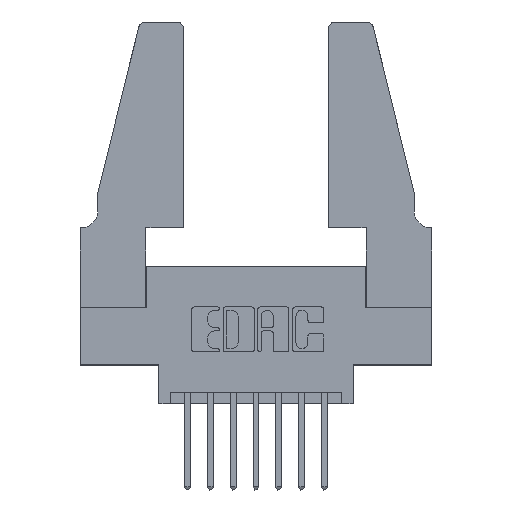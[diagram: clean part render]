
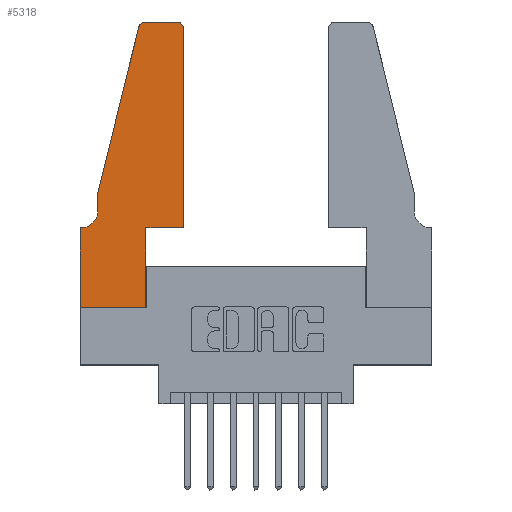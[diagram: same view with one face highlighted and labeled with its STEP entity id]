
A CAD part, top view. The second image highlights one B-rep face of the part: STEP entity #5318.
In plain terms, the highlighted planar face has unit normal (0, 0, 1).
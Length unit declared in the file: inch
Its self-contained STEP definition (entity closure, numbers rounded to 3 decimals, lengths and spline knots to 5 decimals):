
#15 = CARTESIAN_POINT ( 'NONE',  ( 0., 0., 0.37 ) ) ;
#160 = EDGE_CURVE ( 'NONE', #8481, #1776, #9997, .T. ) ;
#842 = CIRCLE ( 'NONE', #3955, 0.03 ) ;
#1019 = ORIENTED_EDGE ( 'NONE', *, *, #10509, .T. ) ;
#1210 = CARTESIAN_POINT ( 'NONE',  ( 0.0755, 0.35, 0.37 ) ) ;
#1450 = ORIENTED_EDGE ( 'NONE', *, *, #7952, .T. ) ;
#1519 = ORIENTED_EDGE ( 'NONE', *, *, #4496, .T. ) ;
#1522 = VECTOR ( 'NONE', #3505, 39.37008 ) ;
#1612 = CARTESIAN_POINT ( 'NONE',  ( 0.2605, 1.25, 0.37 ) ) ;
#1715 = VERTEX_POINT ( 'NONE', #7712 ) ;
#1736 = EDGE_CURVE ( 'NONE', #5225, #1715, #4341, .T. ) ;
#1776 = VERTEX_POINT ( 'NONE', #3939 ) ;
#1782 = VECTOR ( 'NONE', #1790, 39.37008 ) ;
#1790 = DIRECTION ( 'NONE',  ( 0., -1., 0. ) ) ;
#1913 = PLANE ( 'NONE',  #7989 ) ;
#1926 = VERTEX_POINT ( 'NONE', #6098 ) ;
#2149 = ORIENTED_EDGE ( 'NONE', *, *, #1736, .T. ) ;
#2247 = CARTESIAN_POINT ( 'NONE',  ( 0., 0.35, 0.37 ) ) ;
#2248 = CARTESIAN_POINT ( 'NONE',  ( 0.0055, 0.35, 0.37 ) ) ;
#2480 = LINE ( 'NONE', #1612, #10797 ) ;
#2483 = ORIENTED_EDGE ( 'NONE', *, *, #7764, .T. ) ;
#2569 = CARTESIAN_POINT ( 'NONE',  ( 0.2865, 0.35, 0.37 ) ) ;
#2585 = ORIENTED_EDGE ( 'NONE', *, *, #12018, .T. ) ;
#2682 = VERTEX_POINT ( 'NONE', #10618 ) ;
#2702 = CARTESIAN_POINT ( 'NONE',  ( 0.0055, 0.42, 0.37 ) ) ;
#2733 = ORIENTED_EDGE ( 'NONE', *, *, #11453, .T. ) ;
#3236 = ORIENTED_EDGE ( 'NONE', *, *, #4922, .T. ) ;
#3317 = EDGE_LOOP ( 'NONE', ( #8560, #2483, #6055, #1019, #2733, #10747, #2149, #1450, #2585, #3541, #1519, #3236 ) ) ;
#3361 = VERTEX_POINT ( 'NONE', #2248 ) ;
#3505 = DIRECTION ( 'NONE',  ( -0.239, -0.971, 0. ) ) ;
#3541 = ORIENTED_EDGE ( 'NONE', *, *, #160, .T. ) ;
#3655 = VECTOR ( 'NONE', #4179, 39.37008 ) ;
#3939 = CARTESIAN_POINT ( 'NONE',  ( 0.4505, 0.35, 0.37 ) ) ;
#3954 = CARTESIAN_POINT ( 'NONE',  ( 0.4205, 1.25, 0.37 ) ) ;
#3955 = AXIS2_PLACEMENT_3D ( 'NONE', #11658, #5882, #9820 ) ;
#4040 = VECTOR ( 'NONE', #4442, 39.37008 ) ;
#4054 = LINE ( 'NONE', #12157, #10863 ) ;
#4137 = VERTEX_POINT ( 'NONE', #4592 ) ;
#4179 = DIRECTION ( 'NONE',  ( -1., 0., 0. ) ) ;
#4250 = VERTEX_POINT ( 'NONE', #11730 ) ;
#4341 = LINE ( 'NONE', #15, #1782 ) ;
#4442 = DIRECTION ( 'NONE',  ( 1., 0., 0. ) ) ;
#4496 = EDGE_CURVE ( 'NONE', #1776, #2682, #7743, .T. ) ;
#4592 = CARTESIAN_POINT ( 'NONE',  ( 0.0755, 0.42, 0.37 ) ) ;
#4639 = DIRECTION ( 'NONE',  ( 0., 1., 0. ) ) ;
#4673 = EDGE_CURVE ( 'NONE', #6773, #4250, #2480, .T. ) ;
#4731 = CARTESIAN_POINT ( 'NONE',  ( 0.284, 1.22, 0.37 ) ) ;
#4922 = EDGE_CURVE ( 'NONE', #2682, #6773, #842, .T. ) ;
#5225 = VERTEX_POINT ( 'NONE', #2247 ) ;
#5318 = ADVANCED_FACE ( 'NONE', ( #6050 ), #1913, .T. ) ;
#5335 = CARTESIAN_POINT ( 'NONE',  ( 0., 0., 0.37 ) ) ;
#5366 = CARTESIAN_POINT ( 'NONE',  ( 0.0755, 0.5, 0.37 ) ) ;
#5504 = EDGE_CURVE ( 'NONE', #5703, #12047, #11798, .T. ) ;
#5703 = VERTEX_POINT ( 'NONE', #7612 ) ;
#5882 = DIRECTION ( 'NONE',  ( 0., 0., 1. ) ) ;
#6050 = FACE_OUTER_BOUND ( 'NONE', #3317, .T. ) ;
#6055 = ORIENTED_EDGE ( 'NONE', *, *, #5504, .T. ) ;
#6098 = CARTESIAN_POINT ( 'NONE',  ( 0.2865, 0., 0.37 ) ) ;
#6156 = DIRECTION ( 'NONE',  ( 1., 0., 0. ) ) ;
#6416 = AXIS2_PLACEMENT_3D ( 'NONE', #2702, #9450, #10453 ) ;
#6502 = DIRECTION ( 'NONE',  ( 0., 0., 1. ) ) ;
#6531 = LINE ( 'NONE', #7514, #7433 ) ;
#6541 = AXIS2_PLACEMENT_3D ( 'NONE', #4731, #9343, #7278 ) ;
#6546 = DIRECTION ( 'NONE',  ( 0., -1., 0. ) ) ;
#6773 = VERTEX_POINT ( 'NONE', #3954 ) ;
#7278 = DIRECTION ( 'NONE',  ( 1., 0., 0. ) ) ;
#7295 = CARTESIAN_POINT ( 'NONE',  ( 0.0755, 0.5, 0.37 ) ) ;
#7352 = CARTESIAN_POINT ( 'NONE',  ( 0., 0.35, 0.37 ) ) ;
#7433 = VECTOR ( 'NONE', #6546, 39.37008 ) ;
#7514 = CARTESIAN_POINT ( 'NONE',  ( 0.0755, 0.5, 0.37 ) ) ;
#7612 = CARTESIAN_POINT ( 'NONE',  ( 0.25487, 1.22718, 0.37 ) ) ;
#7712 = CARTESIAN_POINT ( 'NONE',  ( 0., 0., 0.37 ) ) ;
#7743 = LINE ( 'NONE', #9422, #12440 ) ;
#7764 = EDGE_CURVE ( 'NONE', #4250, #5703, #8559, .T. ) ;
#7896 = CARTESIAN_POINT ( 'NONE',  ( 0.4505, 0.35, 0.37 ) ) ;
#7952 = EDGE_CURVE ( 'NONE', #1715, #1926, #11731, .T. ) ;
#7989 = AXIS2_PLACEMENT_3D ( 'NONE', #7352, #6502, #6156 ) ;
#8481 = VERTEX_POINT ( 'NONE', #2569 ) ;
#8559 = CIRCLE ( 'NONE', #6541, 0.03 ) ;
#8560 = ORIENTED_EDGE ( 'NONE', *, *, #4673, .T. ) ;
#8761 = VECTOR ( 'NONE', #9913, 39.37008 ) ;
#9343 = DIRECTION ( 'NONE',  ( 0., 0., 1. ) ) ;
#9395 = DIRECTION ( 'NONE',  ( -1., 0., 0. ) ) ;
#9416 = LINE ( 'NONE', #1210, #3655 ) ;
#9422 = CARTESIAN_POINT ( 'NONE',  ( 0.4505, 0.35, 0.37 ) ) ;
#9450 = DIRECTION ( 'NONE',  ( 0., 0., -1. ) ) ;
#9820 = DIRECTION ( 'NONE',  ( 1., 0., 0. ) ) ;
#9913 = DIRECTION ( 'NONE',  ( 1., 0., 0. ) ) ;
#9997 = LINE ( 'NONE', #7896, #8761 ) ;
#10224 = DIRECTION ( 'NONE',  ( 0., 1., 0. ) ) ;
#10453 = DIRECTION ( 'NONE',  ( -1., 0., 0. ) ) ;
#10509 = EDGE_CURVE ( 'NONE', #12047, #4137, #6531, .T. ) ;
#10618 = CARTESIAN_POINT ( 'NONE',  ( 0.4505, 1.22, 0.37 ) ) ;
#10747 = ORIENTED_EDGE ( 'NONE', *, *, #10869, .T. ) ;
#10797 = VECTOR ( 'NONE', #9395, 39.37008 ) ;
#10863 = VECTOR ( 'NONE', #10224, 39.37008 ) ;
#10869 = EDGE_CURVE ( 'NONE', #3361, #5225, #9416, .T. ) ;
#11453 = EDGE_CURVE ( 'NONE', #4137, #3361, #11584, .T. ) ;
#11584 = CIRCLE ( 'NONE', #6416, 0.07 ) ;
#11658 = CARTESIAN_POINT ( 'NONE',  ( 0.4205, 1.22, 0.37 ) ) ;
#11730 = CARTESIAN_POINT ( 'NONE',  ( 0.284, 1.25, 0.37 ) ) ;
#11731 = LINE ( 'NONE', #5335, #4040 ) ;
#11798 = LINE ( 'NONE', #5366, #1522 ) ;
#12018 = EDGE_CURVE ( 'NONE', #1926, #8481, #4054, .T. ) ;
#12047 = VERTEX_POINT ( 'NONE', #7295 ) ;
#12157 = CARTESIAN_POINT ( 'NONE',  ( 0.2865, 0.35, 0.37 ) ) ;
#12440 = VECTOR ( 'NONE', #4639, 39.37008 ) ;
